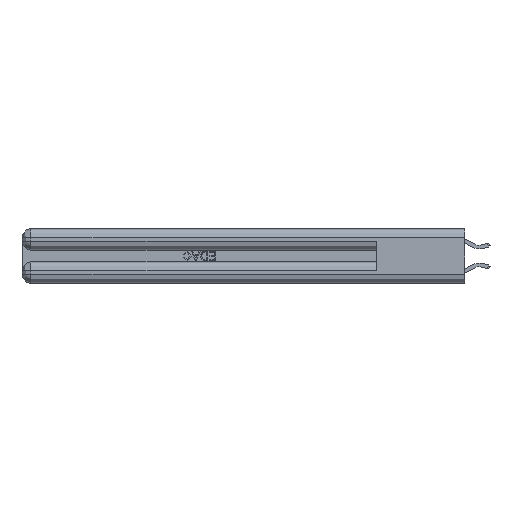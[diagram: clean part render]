
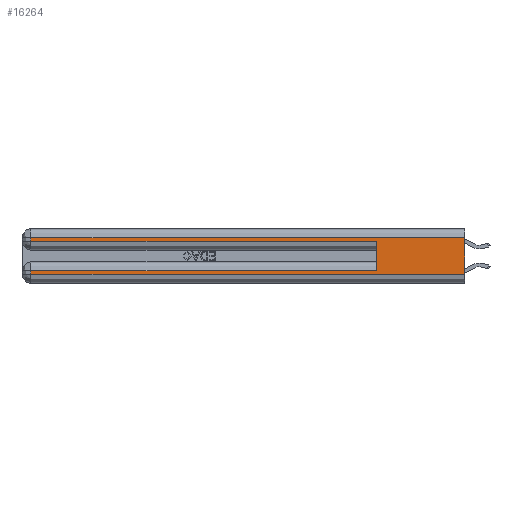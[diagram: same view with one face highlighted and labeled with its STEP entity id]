
A CAD part, left-side view. The second image highlights one B-rep face of the part: STEP entity #16264.
In plain terms, the highlighted planar face has unit normal (-1, 0, 0).
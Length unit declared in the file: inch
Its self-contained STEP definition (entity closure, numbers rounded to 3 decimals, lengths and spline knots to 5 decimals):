
#278 = EDGE_CURVE ( 'NONE', #21361, #3779, #33689, .T. ) ;
#700 = LINE ( 'NONE', #11283, #26909 ) ;
#1312 = CARTESIAN_POINT ( 'NONE',  ( 0., 0.6, 0.145 ) ) ;
#2554 = ORIENTED_EDGE ( 'NONE', *, *, #26109, .T. ) ;
#2671 = CARTESIAN_POINT ( 'NONE',  ( 0., 0., 0.31 ) ) ;
#2702 = DIRECTION ( 'NONE',  ( 0., 0., -1. ) ) ;
#2831 = CARTESIAN_POINT ( 'NONE',  ( 0., 2.94, 0.285 ) ) ;
#3264 = EDGE_CURVE ( 'NONE', #19876, #19802, #23006, .T. ) ;
#3779 = VERTEX_POINT ( 'NONE', #24503 ) ;
#3830 = VECTOR ( 'NONE', #28985, 39.37008 ) ;
#3879 = LINE ( 'NONE', #27645, #5801 ) ;
#4705 = VERTEX_POINT ( 'NONE', #24244 ) ;
#5161 = CARTESIAN_POINT ( 'NONE',  ( 0., 2.94, 0.31 ) ) ;
#5801 = VECTOR ( 'NONE', #14637, 39.37008 ) ;
#6606 = VECTOR ( 'NONE', #9806, 39.37008 ) ;
#6613 = ORIENTED_EDGE ( 'NONE', *, *, #3264, .T. ) ;
#7183 = EDGE_CURVE ( 'NONE', #19802, #4705, #22788, .T. ) ;
#7259 = PLANE ( 'NONE',  #18194 ) ;
#7411 = CARTESIAN_POINT ( 'NONE',  ( 0., 0., 0.06 ) ) ;
#8012 = CARTESIAN_POINT ( 'NONE',  ( 0., 0., 0.285 ) ) ;
#8276 = ORIENTED_EDGE ( 'NONE', *, *, #9236, .F. ) ;
#8368 = LINE ( 'NONE', #14181, #30910 ) ;
#9236 = EDGE_CURVE ( 'NONE', #17576, #4705, #700, .T. ) ;
#9544 = ORIENTED_EDGE ( 'NONE', *, *, #25594, .T. ) ;
#9806 = DIRECTION ( 'NONE',  ( 0., -1., 0. ) ) ;
#10942 = DIRECTION ( 'NONE',  ( 0., 0., -1. ) ) ;
#11283 = CARTESIAN_POINT ( 'NONE',  ( 0., 0., 0.37 ) ) ;
#12617 = ORIENTED_EDGE ( 'NONE', *, *, #26517, .F. ) ;
#13630 = CARTESIAN_POINT ( 'NONE',  ( 0., 2.94, 0.06 ) ) ;
#14181 = CARTESIAN_POINT ( 'NONE',  ( 0., 0., 0.085 ) ) ;
#14535 = VECTOR ( 'NONE', #18921, 39.37008 ) ;
#14637 = DIRECTION ( 'NONE',  ( 0., 1., 0. ) ) ;
#15455 = DIRECTION ( 'NONE',  ( 0., 0., -1. ) ) ;
#15493 = CARTESIAN_POINT ( 'NONE',  ( 0., 2.94, 0.37 ) ) ;
#16264 = ADVANCED_FACE ( 'NONE', ( #25202 ), #7259, .F. ) ;
#16849 = LINE ( 'NONE', #1312, #14535 ) ;
#17165 = CARTESIAN_POINT ( 'NONE',  ( 0., 2.94, 0.085 ) ) ;
#17576 = VERTEX_POINT ( 'NONE', #2671 ) ;
#18194 = AXIS2_PLACEMENT_3D ( 'NONE', #33109, #33446, #15455 ) ;
#18885 = VECTOR ( 'NONE', #2702, 39.37008 ) ;
#18921 = DIRECTION ( 'NONE',  ( 0., 0., 1. ) ) ;
#19029 = LINE ( 'NONE', #31551, #3830 ) ;
#19076 = CARTESIAN_POINT ( 'NONE',  ( 0., 0.6, 0.085 ) ) ;
#19802 = VERTEX_POINT ( 'NONE', #13630 ) ;
#19876 = VERTEX_POINT ( 'NONE', #17165 ) ;
#20176 = VECTOR ( 'NONE', #25620, 39.37008 ) ;
#20253 = EDGE_LOOP ( 'NONE', ( #8276, #2554, #21903, #20336, #12617, #9544, #6613, #30631 ) ) ;
#20336 = ORIENTED_EDGE ( 'NONE', *, *, #278, .T. ) ;
#21361 = VERTEX_POINT ( 'NONE', #2831 ) ;
#21903 = ORIENTED_EDGE ( 'NONE', *, *, #30966, .T. ) ;
#22788 = LINE ( 'NONE', #7411, #6606 ) ;
#23006 = LINE ( 'NONE', #15493, #18885 ) ;
#23084 = VERTEX_POINT ( 'NONE', #19076 ) ;
#24244 = CARTESIAN_POINT ( 'NONE',  ( 0., 0., 0.06 ) ) ;
#24503 = CARTESIAN_POINT ( 'NONE',  ( 0., 0.6, 0.285 ) ) ;
#25202 = FACE_OUTER_BOUND ( 'NONE', #20253, .T. ) ;
#25594 = EDGE_CURVE ( 'NONE', #23084, #19876, #8368, .T. ) ;
#25620 = DIRECTION ( 'NONE',  ( 0., -1., 0. ) ) ;
#26109 = EDGE_CURVE ( 'NONE', #17576, #32357, #3879, .T. ) ;
#26517 = EDGE_CURVE ( 'NONE', #23084, #3779, #16849, .T. ) ;
#26909 = VECTOR ( 'NONE', #10942, 39.37008 ) ;
#27193 = DIRECTION ( 'NONE',  ( 0., 1., 0. ) ) ;
#27645 = CARTESIAN_POINT ( 'NONE',  ( 0., 0., 0.31 ) ) ;
#28985 = DIRECTION ( 'NONE',  ( 0., 0., -1. ) ) ;
#30631 = ORIENTED_EDGE ( 'NONE', *, *, #7183, .T. ) ;
#30910 = VECTOR ( 'NONE', #27193, 39.37008 ) ;
#30966 = EDGE_CURVE ( 'NONE', #32357, #21361, #19029, .T. ) ;
#31551 = CARTESIAN_POINT ( 'NONE',  ( 0., 2.94, 0.37 ) ) ;
#32357 = VERTEX_POINT ( 'NONE', #5161 ) ;
#33109 = CARTESIAN_POINT ( 'NONE',  ( 0., 0., 0.37 ) ) ;
#33446 = DIRECTION ( 'NONE',  ( 1., 0., 0. ) ) ;
#33689 = LINE ( 'NONE', #8012, #20176 ) ;
